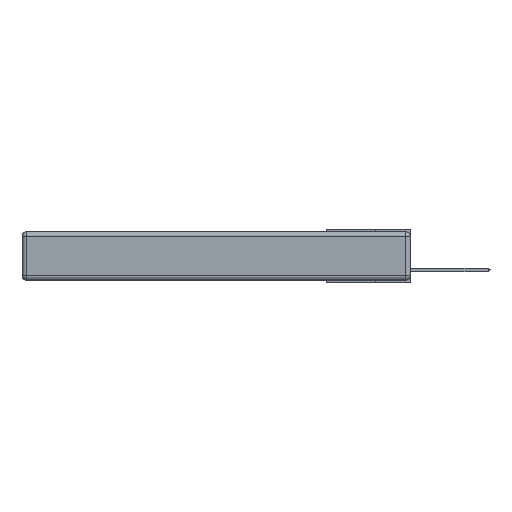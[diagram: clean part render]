
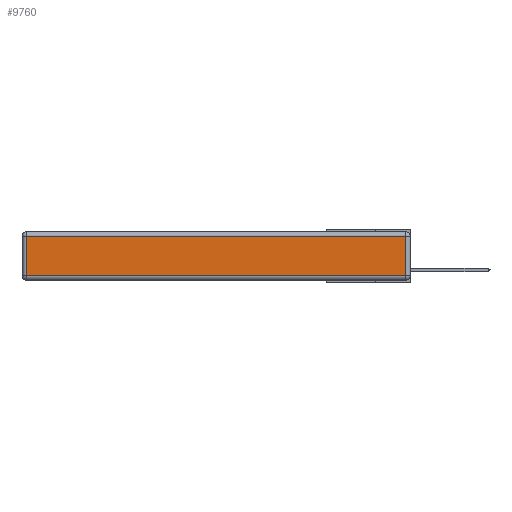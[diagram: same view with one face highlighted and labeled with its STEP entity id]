
A CAD part, left-side view. The second image highlights one B-rep face of the part: STEP entity #9760.
In plain terms, the highlighted planar face has unit normal (-1, 0, 0).
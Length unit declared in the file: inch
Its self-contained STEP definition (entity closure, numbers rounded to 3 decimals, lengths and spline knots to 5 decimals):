
#2414 = DIRECTION ( 'NONE',  ( 0., 0., 1. ) ) ;
#2521 = LINE ( 'NONE', #18861, #14794 ) ;
#2768 = DIRECTION ( 'NONE',  ( 0., 1., 0. ) ) ;
#2833 = VECTOR ( 'NONE', #21043, 39.37008 ) ;
#3655 = EDGE_CURVE ( 'NONE', #18778, #5046, #2521, .T. ) ;
#5000 = CARTESIAN_POINT ( 'NONE',  ( 0., 0.03, -0.313 ) ) ;
#5046 = VERTEX_POINT ( 'NONE', #17680 ) ;
#5050 = EDGE_LOOP ( 'NONE', ( #6756, #7001, #17725, #9388 ) ) ;
#5823 = EDGE_CURVE ( 'NONE', #5046, #10683, #6848, .T. ) ;
#5969 = CARTESIAN_POINT ( 'NONE',  ( 0., 0., -0.343 ) ) ;
#6756 = ORIENTED_EDGE ( 'NONE', *, *, #11274, .T. ) ;
#6848 = LINE ( 'NONE', #10589, #17983 ) ;
#7001 = ORIENTED_EDGE ( 'NONE', *, *, #19922, .T. ) ;
#7158 = LINE ( 'NONE', #8063, #2833 ) ;
#8063 = CARTESIAN_POINT ( 'NONE',  ( 0., 0., -0.313 ) ) ;
#9388 = ORIENTED_EDGE ( 'NONE', *, *, #5823, .T. ) ;
#9673 = CARTESIAN_POINT ( 'NONE',  ( 0., 2.72, -0.313 ) ) ;
#9760 = ADVANCED_FACE ( 'NONE', ( #11008 ), #12215, .T. ) ;
#10589 = CARTESIAN_POINT ( 'NONE',  ( 0., 2.72, -0.343 ) ) ;
#10683 = VERTEX_POINT ( 'NONE', #9673 ) ;
#10734 = VERTEX_POINT ( 'NONE', #5000 ) ;
#11008 = FACE_OUTER_BOUND ( 'NONE', #5050, .T. ) ;
#11097 = AXIS2_PLACEMENT_3D ( 'NONE', #5969, #18674, #2414 ) ;
#11274 = EDGE_CURVE ( 'NONE', #10683, #10734, #7158, .T. ) ;
#11628 = LINE ( 'NONE', #18709, #14616 ) ;
#12210 = DIRECTION ( 'NONE',  ( 0., 0., -1. ) ) ;
#12215 = PLANE ( 'NONE',  #11097 ) ;
#12259 = DIRECTION ( 'NONE',  ( 0., 0., 1. ) ) ;
#14616 = VECTOR ( 'NONE', #12259, 39.37008 ) ;
#14794 = VECTOR ( 'NONE', #2768, 39.37008 ) ;
#16000 = CARTESIAN_POINT ( 'NONE',  ( 0., 0.03, -0.03 ) ) ;
#17680 = CARTESIAN_POINT ( 'NONE',  ( 0., 2.72, -0.03 ) ) ;
#17725 = ORIENTED_EDGE ( 'NONE', *, *, #3655, .T. ) ;
#17983 = VECTOR ( 'NONE', #12210, 39.37008 ) ;
#18674 = DIRECTION ( 'NONE',  ( -1., 0., 0. ) ) ;
#18709 = CARTESIAN_POINT ( 'NONE',  ( 0., 0.03, -0.343 ) ) ;
#18778 = VERTEX_POINT ( 'NONE', #16000 ) ;
#18861 = CARTESIAN_POINT ( 'NONE',  ( 0., 2.75, -0.03 ) ) ;
#19922 = EDGE_CURVE ( 'NONE', #10734, #18778, #11628, .T. ) ;
#21043 = DIRECTION ( 'NONE',  ( 0., -1., 0. ) ) ;
